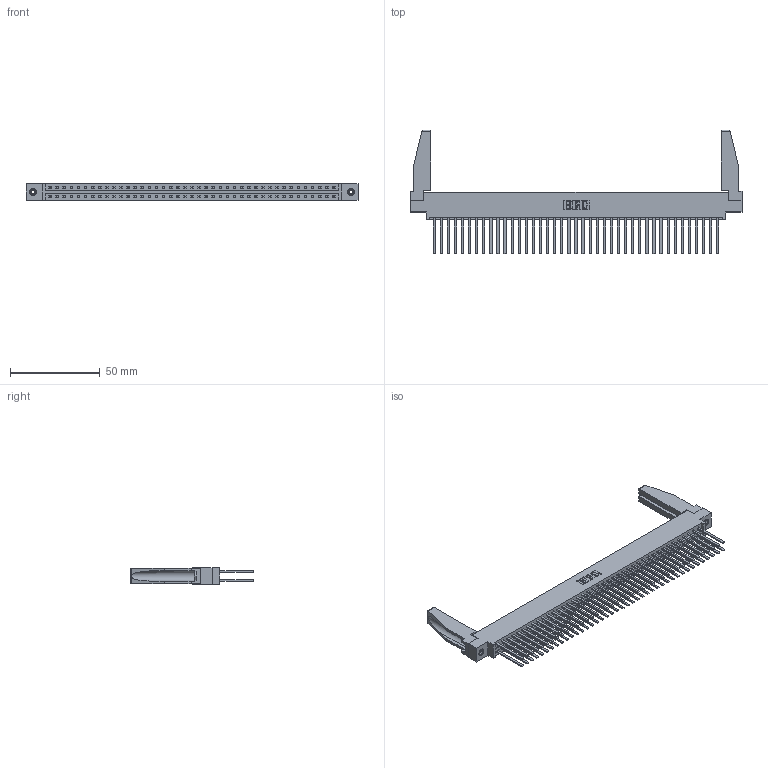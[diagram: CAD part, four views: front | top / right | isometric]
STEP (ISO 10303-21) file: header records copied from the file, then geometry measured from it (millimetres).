
FILE_DESCRIPTION (( 'STEP AP203' ), '1' );
FILE_NAME ('337-082-544-878.STEP', '2019-10-15T17:25:14', ( '' ), ( '' ), 'SwSTEP 2.0', 'SolidWorks 2016', '' );
FILE_SCHEMA (( 'CONFIG_CONTROL_DESIGN' ));
Length unit declared in the file: inch
Products named in the file (5): 337 Part_0.170 Offset - 0.156 Dia-TI; 337-082-544-878; 345-250-001_345-250-001-102; 307-220-078; 345-292-001_345-293-144
Assembly tree (87 placements, depth 2):
  337-082-544-878
    337 Part_0.170 Offset - 0.156 Dia-TI
    345-292-001_345-293-144  x82
    345-250-001_345-250-001-102  x2
    307-220-078  x2
Bounding box: 185.47 x 69.09 x 9.4 mm (x, y, z)
Volume: 24558.4 mm3; surface area: 30932.5 mm2
Topology: 87 solids, 87 shells, 4184 faces, 12379 edges, 8134 vertices
Faces by surface type: plane 2946, cylinder 1222, cone 12, torus 4
Entity records: 34306 total; most frequent: CARTESIAN_POINT 5780, ORIENTED_EDGE 5672, DIRECTION 4920, EDGE_CURVE 2836, VECTOR 2674, LINE 2674, VERTEX_POINT 1884, AXIS2_PLACEMENT_3D 1123
